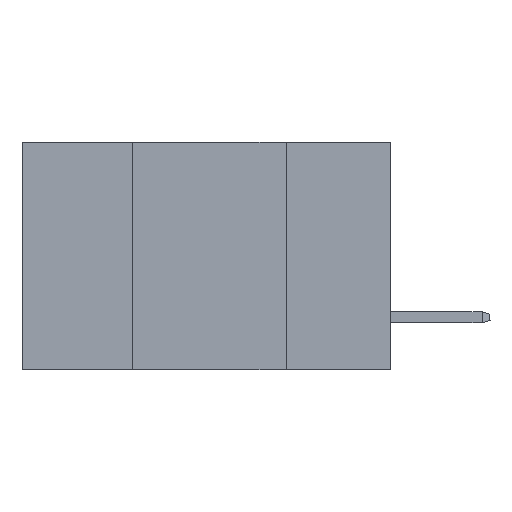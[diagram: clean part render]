
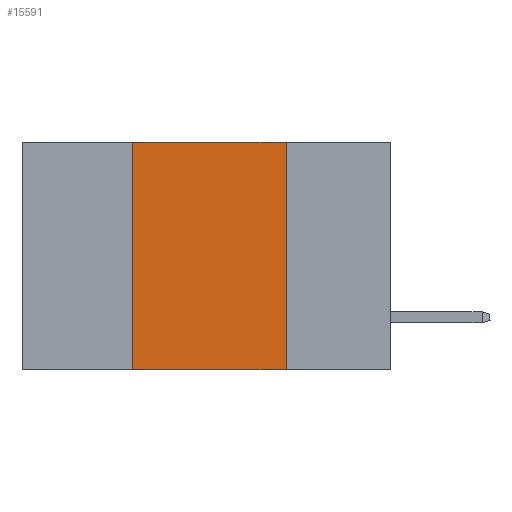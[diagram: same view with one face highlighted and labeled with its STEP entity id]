
A CAD part, left-side view. The second image highlights one B-rep face of the part: STEP entity #15591.
In plain terms, the highlighted planar face has unit normal (-1, 0, 0).
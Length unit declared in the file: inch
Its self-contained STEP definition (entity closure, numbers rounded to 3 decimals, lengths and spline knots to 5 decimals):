
#1905 = EDGE_CURVE ( 'NONE', #13280, #34405, #30190, .T. ) ;
#1943 = CARTESIAN_POINT ( 'NONE',  ( 0., 0.42, 0. ) ) ;
#2103 = VERTEX_POINT ( 'NONE', #1943 ) ;
#3574 = LINE ( 'NONE', #14904, #24092 ) ;
#4075 = FACE_OUTER_BOUND ( 'NONE', #24589, .T. ) ;
#4821 = DIRECTION ( 'NONE',  ( 0., 0., 1. ) ) ;
#5520 = VECTOR ( 'NONE', #4821, 39.37008 ) ;
#5758 = VERTEX_POINT ( 'NONE', #35228 ) ;
#5898 = DIRECTION ( 'NONE',  ( 0., 0., -1. ) ) ;
#6215 = EDGE_CURVE ( 'NONE', #5758, #2103, #20317, .T. ) ;
#9591 = CARTESIAN_POINT ( 'NONE',  ( 0., 0.42, 0. ) ) ;
#11215 = ORIENTED_EDGE ( 'NONE', *, *, #19250, .T. ) ;
#11321 = CARTESIAN_POINT ( 'NONE',  ( 0., 0.17, 0. ) ) ;
#11877 = ORIENTED_EDGE ( 'NONE', *, *, #1905, .F. ) ;
#13222 = VECTOR ( 'NONE', #26533, 39.37008 ) ;
#13280 = VERTEX_POINT ( 'NONE', #16834 ) ;
#14904 = CARTESIAN_POINT ( 'NONE',  ( 0., 0.6, 0. ) ) ;
#15591 = ADVANCED_FACE ( 'NONE', ( #4075 ), #20022, .F. ) ;
#16200 = ORIENTED_EDGE ( 'NONE', *, *, #6215, .F. ) ;
#16834 = CARTESIAN_POINT ( 'NONE',  ( 0., 0.17, 0. ) ) ;
#16950 = CARTESIAN_POINT ( 'NONE',  ( 0., 0.6, 0. ) ) ;
#19250 = EDGE_CURVE ( 'NONE', #5758, #34405, #21536, .T. ) ;
#19408 = AXIS2_PLACEMENT_3D ( 'NONE', #16950, #33463, #5898 ) ;
#19416 = DIRECTION ( 'NONE',  ( 0., 0., -1. ) ) ;
#20022 = PLANE ( 'NONE',  #19408 ) ;
#20317 = LINE ( 'NONE', #9591, #5520 ) ;
#21536 = LINE ( 'NONE', #35069, #13222 ) ;
#23628 = VECTOR ( 'NONE', #19416, 39.37008 ) ;
#24092 = VECTOR ( 'NONE', #35338, 39.37008 ) ;
#24589 = EDGE_LOOP ( 'NONE', ( #11877, #29987, #16200, #11215 ) ) ;
#25303 = EDGE_CURVE ( 'NONE', #2103, #13280, #3574, .T. ) ;
#26533 = DIRECTION ( 'NONE',  ( 0., -1., 0. ) ) ;
#29987 = ORIENTED_EDGE ( 'NONE', *, *, #25303, .F. ) ;
#30190 = LINE ( 'NONE', #11321, #23628 ) ;
#33463 = DIRECTION ( 'NONE',  ( 1., 0., 0. ) ) ;
#34246 = CARTESIAN_POINT ( 'NONE',  ( 0., 0.17, -0.37 ) ) ;
#34405 = VERTEX_POINT ( 'NONE', #34246 ) ;
#35069 = CARTESIAN_POINT ( 'NONE',  ( 0., 0.6, -0.37 ) ) ;
#35228 = CARTESIAN_POINT ( 'NONE',  ( 0., 0.42, -0.37 ) ) ;
#35338 = DIRECTION ( 'NONE',  ( 0., -1., 0. ) ) ;
